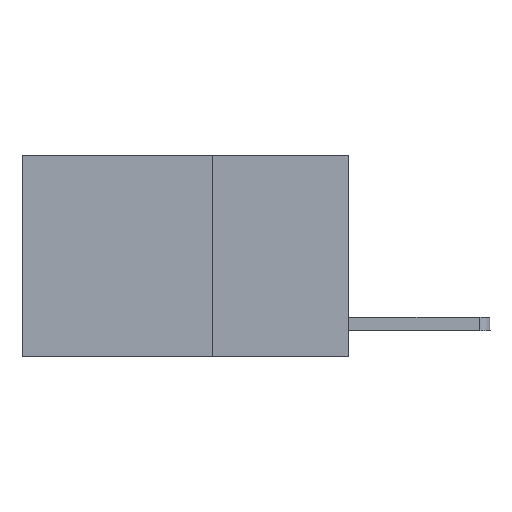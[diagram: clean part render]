
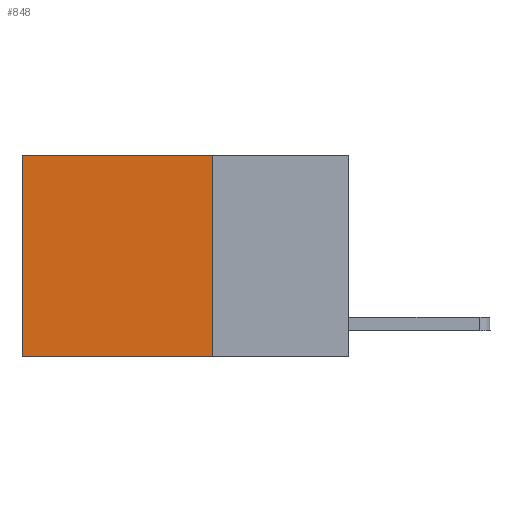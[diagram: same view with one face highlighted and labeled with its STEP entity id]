
A CAD part, left-side view. The second image highlights one B-rep face of the part: STEP entity #848.
In plain terms, the highlighted planar face has unit normal (-1, 0, 0).
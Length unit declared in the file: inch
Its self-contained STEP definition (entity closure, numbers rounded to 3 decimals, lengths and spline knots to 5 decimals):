
#292 = ORIENTED_EDGE ( 'NONE', *, *, #6618, .T. ) ;
#296 = PLANE ( 'NONE',  #4825 ) ;
#717 = DIRECTION ( 'NONE',  ( 0., 0., -1. ) ) ;
#848 = ADVANCED_FACE ( 'NONE', ( #8091 ), #296, .F. ) ;
#908 = EDGE_CURVE ( 'NONE', #4042, #8413, #4306, .T. ) ;
#1365 = CARTESIAN_POINT ( 'NONE',  ( 0.2625, 0.25, -0.37 ) ) ;
#1484 = LINE ( 'NONE', #2080, #1863 ) ;
#1523 = CARTESIAN_POINT ( 'NONE',  ( 0.2625, 0.25, 0. ) ) ;
#1615 = CARTESIAN_POINT ( 'NONE',  ( 0.2625, 0.6, -0.37 ) ) ;
#1863 = VECTOR ( 'NONE', #2031, 39.37008 ) ;
#1877 = CARTESIAN_POINT ( 'NONE',  ( 0.2625, 0.25, 0. ) ) ;
#2031 = DIRECTION ( 'NONE',  ( 0., 0., -1. ) ) ;
#2080 = CARTESIAN_POINT ( 'NONE',  ( 0.2625, 0.25, 0. ) ) ;
#2542 = DIRECTION ( 'NONE',  ( 0., 1., 0. ) ) ;
#2631 = LINE ( 'NONE', #5902, #4786 ) ;
#2752 = CARTESIAN_POINT ( 'NONE',  ( 0.2625, 0.6, 0. ) ) ;
#2849 = CARTESIAN_POINT ( 'NONE',  ( 0.2625, 0.25, -0.37 ) ) ;
#2894 = DIRECTION ( 'NONE',  ( 0., 0., -1. ) ) ;
#4042 = VERTEX_POINT ( 'NONE', #1365 ) ;
#4186 = ORIENTED_EDGE ( 'NONE', *, *, #7513, .T. ) ;
#4269 = DIRECTION ( 'NONE',  ( 1., 0., 0. ) ) ;
#4306 = LINE ( 'NONE', #2849, #8379 ) ;
#4577 = EDGE_CURVE ( 'NONE', #5268, #4042, #1484, .T. ) ;
#4786 = VECTOR ( 'NONE', #717, 39.37008 ) ;
#4825 = AXIS2_PLACEMENT_3D ( 'NONE', #1523, #4269, #2894 ) ;
#5268 = VERTEX_POINT ( 'NONE', #1877 ) ;
#5723 = ORIENTED_EDGE ( 'NONE', *, *, #908, .F. ) ;
#5902 = CARTESIAN_POINT ( 'NONE',  ( 0.2625, 0.6, 0. ) ) ;
#6206 = DIRECTION ( 'NONE',  ( 0., 1., 0. ) ) ;
#6464 = LINE ( 'NONE', #8420, #6842 ) ;
#6525 = ORIENTED_EDGE ( 'NONE', *, *, #4577, .F. ) ;
#6581 = VERTEX_POINT ( 'NONE', #2752 ) ;
#6618 = EDGE_CURVE ( 'NONE', #5268, #6581, #6464, .T. ) ;
#6842 = VECTOR ( 'NONE', #2542, 39.37008 ) ;
#7101 = EDGE_LOOP ( 'NONE', ( #4186, #5723, #6525, #292 ) ) ;
#7513 = EDGE_CURVE ( 'NONE', #6581, #8413, #2631, .T. ) ;
#8091 = FACE_OUTER_BOUND ( 'NONE', #7101, .T. ) ;
#8379 = VECTOR ( 'NONE', #6206, 39.37008 ) ;
#8413 = VERTEX_POINT ( 'NONE', #1615 ) ;
#8420 = CARTESIAN_POINT ( 'NONE',  ( 0.2625, 0.25, 0. ) ) ;
